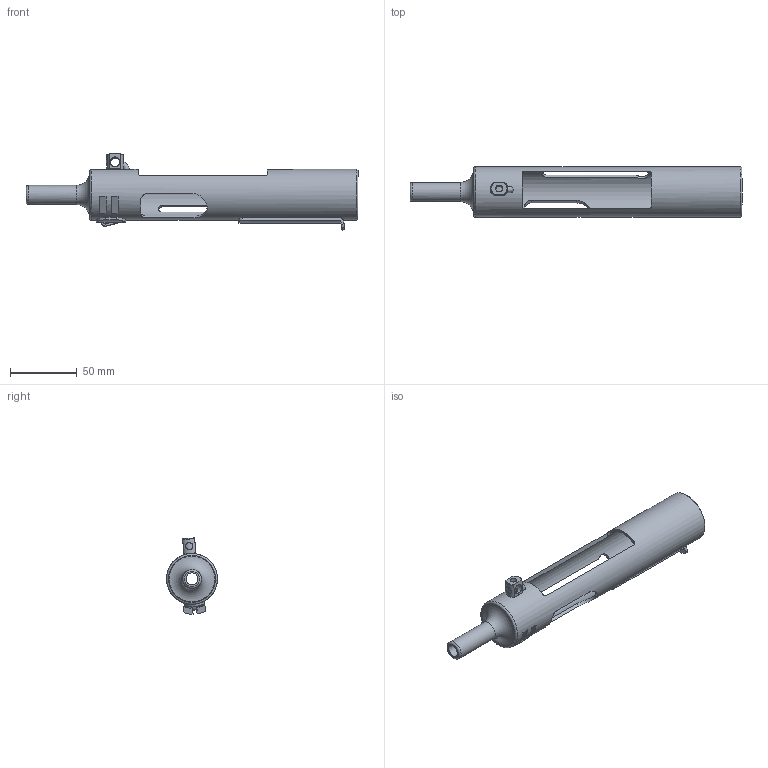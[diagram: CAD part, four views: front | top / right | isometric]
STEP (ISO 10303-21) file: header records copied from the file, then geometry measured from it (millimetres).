
FILE_DESCRIPTION(/* description */ (''),/* implementation_level */ '2;1');
FILE_NAME(/* name */ 'AB10.step',/* time_stamp */ '2025-06-07T20:19:29-04:00',/* author */ (''),/* organization */ (''),/* preprocessor_version */ 'ST-DEVELOPER v20.1',/* originating_system */ 'Autodesk Translation Framework v14.10.0.0',/* authorisation */ '');
FILE_SCHEMA (('AUTOMOTIVE_DESIGN { 1 0 10303 214 3 1 1 }'));
Length unit declared in the file: millimetre
Products named in the file (1): Mock Up Tec 9
Bounding box: 248.2 x 38.1 x 56.95 mm (x, y, z)
Volume: 49725.1 mm3; surface area: 46891.8 mm2
Topology: 5 solids, 5 shells, 107 faces, 272 edges, 181 vertices
Faces by surface type: plane 48, cylinder 39, bspline 11, cone 5, torus 4
Full cylindrical faces by diameter (mm): 5 x2, 5.5 x1, 7 x1, 8 x1, 9 x1, 14.2 x1, 34.1 x1, 38.1 x1
Entity records: 5316 total; most frequent: CARTESIAN_POINT 2746, ORIENTED_EDGE 544, DIRECTION 473, EDGE_CURVE 272, VERTEX_POINT 181, AXIS2_PLACEMENT_3D 173, EDGE_LOOP 131, LINE 127
